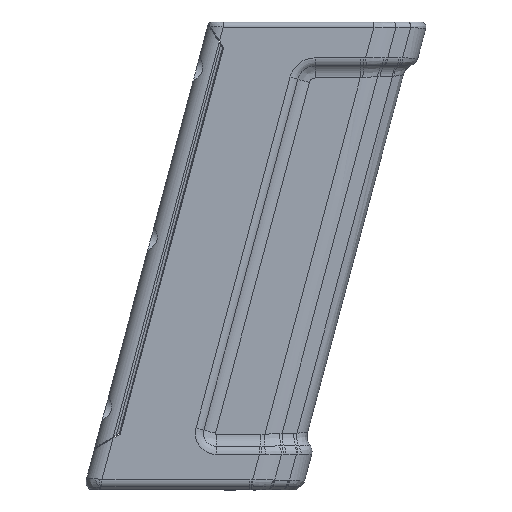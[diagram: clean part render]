
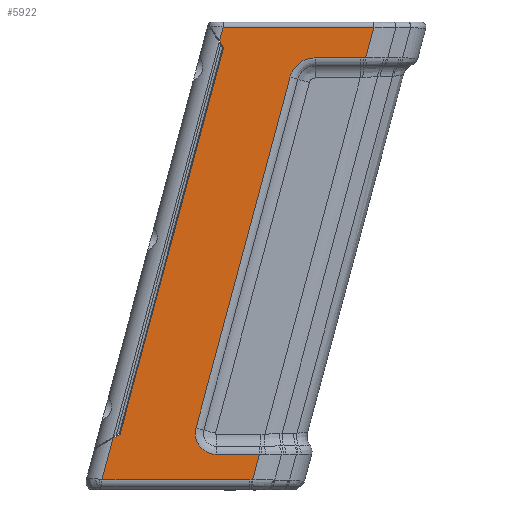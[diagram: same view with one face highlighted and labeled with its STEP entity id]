
A CAD part, left-side view. The second image highlights one B-rep face of the part: STEP entity #5922.
In plain terms, the highlighted planar face has unit normal (-1, 0, 0).
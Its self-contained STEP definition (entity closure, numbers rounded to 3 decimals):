
#297=PLANE('',#6416);
#440=FACE_OUTER_BOUND('',#836,.T.);
#836=EDGE_LOOP('',(#4337,#4338,#4339,#4340,#4341,#4342,#4343,#4344,#4345,
#4346,#4347,#4348,#4349,#4350,#4351,#4352,#4353,#4354));
#1217=LINE('',#9080,#1559);
#1229=LINE('',#9156,#1571);
#1238=LINE('',#9196,#1580);
#1246=LINE('',#9251,#1588);
#1247=LINE('',#9253,#1589);
#1248=LINE('',#9265,#1590);
#1249=LINE('',#9267,#1591);
#1250=LINE('',#9271,#1592);
#1251=LINE('',#9275,#1593);
#1252=LINE('',#9287,#1594);
#1253=LINE('',#9288,#1595);
#1254=LINE('',#9289,#1596);
#1559=VECTOR('',#7221,10.);
#1571=VECTOR('',#7247,10.);
#1580=VECTOR('',#7264,10.);
#1588=VECTOR('',#7294,10.);
#1589=VECTOR('',#7295,10.);
#1590=VECTOR('',#7296,10.);
#1591=VECTOR('',#7297,10.);
#1592=VECTOR('',#7300,10.);
#1593=VECTOR('',#7303,10.);
#1594=VECTOR('',#7304,10.);
#1595=VECTOR('',#7305,10.);
#1596=VECTOR('',#7306,10.);
#1888=CIRCLE('',#6417,4.172);
#1889=CIRCLE('',#6418,5.172);
#2124=B_SPLINE_CURVE_WITH_KNOTS('',3,(#9255,#9256,#9257,#9258),
 .UNSPECIFIED.,.F.,.F.,(4,4),(0.,0.029),.UNSPECIFIED.);
#2125=B_SPLINE_CURVE_WITH_KNOTS('',3,(#9260,#9261,#9262,#9263),
 .UNSPECIFIED.,.F.,.F.,(4,4),(0.,0.027),.UNSPECIFIED.);
#2126=B_SPLINE_CURVE_WITH_KNOTS('',3,(#9277,#9278,#9279,#9280),
 .UNSPECIFIED.,.F.,.F.,(4,4),(-0.063,0.),.UNSPECIFIED.);
#2127=B_SPLINE_CURVE_WITH_KNOTS('',3,(#9282,#9283,#9284,#9285),
 .UNSPECIFIED.,.F.,.F.,(4,4),(-0.045,0.),
 .UNSPECIFIED.);
#2499=VERTEX_POINT('',#9077);
#2500=VERTEX_POINT('',#9079);
#2518=VERTEX_POINT('',#9155);
#2529=VERTEX_POINT('',#9195);
#2538=VERTEX_POINT('',#9244);
#2540=VERTEX_POINT('',#9250);
#2541=VERTEX_POINT('',#9252);
#2542=VERTEX_POINT('',#9254);
#2543=VERTEX_POINT('',#9259);
#2544=VERTEX_POINT('',#9264);
#2545=VERTEX_POINT('',#9266);
#2546=VERTEX_POINT('',#9268);
#2547=VERTEX_POINT('',#9270);
#2548=VERTEX_POINT('',#9272);
#2549=VERTEX_POINT('',#9274);
#2550=VERTEX_POINT('',#9276);
#2551=VERTEX_POINT('',#9281);
#2552=VERTEX_POINT('',#9286);
#3144=EDGE_CURVE('',#2500,#2499,#1217,.T.);
#3165=EDGE_CURVE('',#2518,#2500,#1229,.T.);
#3178=EDGE_CURVE('',#2499,#2529,#1238,.F.);
#3194=EDGE_CURVE('',#2540,#2529,#1246,.T.);
#3195=EDGE_CURVE('',#2541,#2540,#1247,.T.);
#3196=EDGE_CURVE('',#2542,#2541,#2124,.T.);
#3197=EDGE_CURVE('',#2543,#2542,#2125,.T.);
#3198=EDGE_CURVE('',#2544,#2543,#1248,.T.);
#3199=EDGE_CURVE('',#2545,#2544,#1249,.T.);
#3200=EDGE_CURVE('',#2546,#2545,#1888,.T.);
#3201=EDGE_CURVE('',#2547,#2546,#1250,.T.);
#3202=EDGE_CURVE('',#2548,#2547,#1889,.T.);
#3203=EDGE_CURVE('',#2549,#2548,#1251,.T.);
#3204=EDGE_CURVE('',#2550,#2549,#2126,.T.);
#3205=EDGE_CURVE('',#2551,#2550,#2127,.T.);
#3206=EDGE_CURVE('',#2552,#2551,#1252,.T.);
#3207=EDGE_CURVE('',#2538,#2552,#1253,.T.);
#3208=EDGE_CURVE('',#2518,#2538,#1254,.T.);
#4337=ORIENTED_EDGE('',*,*,#3165,.T.);
#4338=ORIENTED_EDGE('',*,*,#3144,.T.);
#4339=ORIENTED_EDGE('',*,*,#3178,.T.);
#4340=ORIENTED_EDGE('',*,*,#3194,.F.);
#4341=ORIENTED_EDGE('',*,*,#3195,.F.);
#4342=ORIENTED_EDGE('',*,*,#3196,.F.);
#4343=ORIENTED_EDGE('',*,*,#3197,.F.);
#4344=ORIENTED_EDGE('',*,*,#3198,.F.);
#4345=ORIENTED_EDGE('',*,*,#3199,.F.);
#4346=ORIENTED_EDGE('',*,*,#3200,.F.);
#4347=ORIENTED_EDGE('',*,*,#3201,.F.);
#4348=ORIENTED_EDGE('',*,*,#3202,.F.);
#4349=ORIENTED_EDGE('',*,*,#3203,.F.);
#4350=ORIENTED_EDGE('',*,*,#3204,.F.);
#4351=ORIENTED_EDGE('',*,*,#3205,.F.);
#4352=ORIENTED_EDGE('',*,*,#3206,.F.);
#4353=ORIENTED_EDGE('',*,*,#3207,.F.);
#4354=ORIENTED_EDGE('',*,*,#3208,.F.);
#5922=ADVANCED_FACE('',(#440),#297,.F.);
#6416=AXIS2_PLACEMENT_3D('',#9249,#7292,#7293);
#6417=AXIS2_PLACEMENT_3D('',#9269,#7298,#7299);
#6418=AXIS2_PLACEMENT_3D('',#9273,#7301,#7302);
#7221=DIRECTION('',(0.,0.259,-0.966));
#7247=DIRECTION('',(0.,-0.537,-0.844));
#7264=DIRECTION('',(0.,-0.86,0.51));
#7292=DIRECTION('center_axis',(1.,0.,0.));
#7293=DIRECTION('ref_axis',(0.,1.,0.));
#7294=DIRECTION('',(0.,-0.259,0.966));
#7295=DIRECTION('',(0.,1.,0.));
#7296=DIRECTION('',(0.,0.259,-0.966));
#7297=DIRECTION('',(0.,-1.,0.));
#7298=DIRECTION('center_axis',(-1.,0.,0.));
#7299=DIRECTION('ref_axis',(0.,0.793,-0.609));
#7300=DIRECTION('',(0.,0.259,-0.966));
#7301=DIRECTION('center_axis',(-1.,0.,0.));
#7302=DIRECTION('ref_axis',(0.,0.609,0.793));
#7303=DIRECTION('',(0.,1.,0.));
#7304=DIRECTION('',(0.,0.259,-0.966));
#7305=DIRECTION('',(0.,-1.,0.));
#7306=DIRECTION('',(0.,-0.259,0.966));
#9077=CARTESIAN_POINT('',(8.281,19.826,-74.034));
#9079=CARTESIAN_POINT('',(8.281,-0.788,2.901));
#9080=CARTESIAN_POINT('',(8.281,11.023,-41.18));
#9155=CARTESIAN_POINT('',(8.281,0.048,4.215));
#9156=CARTESIAN_POINT('',(8.281,-2.855,-0.348));
#9195=CARTESIAN_POINT('',(8.281,21.239,-74.872));
#9196=CARTESIAN_POINT('',(8.281,1.91,-63.414));
#9244=CARTESIAN_POINT('',(8.281,-0.689,6.965));
#9249=CARTESIAN_POINT('Origin',(8.281,2.424,-8.271));
#9250=CARTESIAN_POINT('',(8.281,23.442,-83.093));
#9251=CARTESIAN_POINT('',(8.281,3.465,-8.538));
#9252=CARTESIAN_POINT('',(8.281,-6.,-83.093));
#9253=CARTESIAN_POINT('',(8.281,-2.868,-83.093));
#9254=CARTESIAN_POINT('',(8.281,-6.289,-83.09));
#9255=CARTESIAN_POINT('Ctrl Pts',(8.281,-6.289,-83.09));
#9256=CARTESIAN_POINT('Ctrl Pts',(8.281,-6.192,-83.092));
#9257=CARTESIAN_POINT('Ctrl Pts',(8.281,-6.096,-83.093));
#9258=CARTESIAN_POINT('Ctrl Pts',(8.281,-6.,-83.093));
#9259=CARTESIAN_POINT('',(8.281,-6.56,-83.08));
#9260=CARTESIAN_POINT('Ctrl Pts',(8.281,-6.56,-83.08));
#9261=CARTESIAN_POINT('Ctrl Pts',(8.281,-6.47,-83.085));
#9262=CARTESIAN_POINT('Ctrl Pts',(8.281,-6.379,-83.089));
#9263=CARTESIAN_POINT('Ctrl Pts',(8.281,-6.289,-83.09));
#9264=CARTESIAN_POINT('',(8.281,-7.897,-78.093));
#9265=CARTESIAN_POINT('',(8.281,-28.055,-2.863));
#9266=CARTESIAN_POINT('',(8.281,0.694,-78.093));
#9267=CARTESIAN_POINT('',(8.281,-2.358,-78.093));
#9268=CARTESIAN_POINT('',(8.281,4.723,-72.841));
#9269=CARTESIAN_POINT('Origin',(8.281,0.694,-73.921));
#9270=CARTESIAN_POINT('',(8.281,-13.988,-3.011));
#9271=CARTESIAN_POINT('',(8.281,-13.251,-5.762));
#9272=CARTESIAN_POINT('',(8.281,-18.983,0.822));
#9273=CARTESIAN_POINT('Origin',(8.281,-18.983,-4.349));
#9274=CARTESIAN_POINT('',(8.281,-27.97,0.822));
#9275=CARTESIAN_POINT('',(8.281,-2.358,0.822));
#9276=CARTESIAN_POINT('',(8.281,-28.602,0.832));
#9277=CARTESIAN_POINT('Ctrl Pts',(8.281,-28.602,0.832));
#9278=CARTESIAN_POINT('Ctrl Pts',(8.281,-28.391,0.826));
#9279=CARTESIAN_POINT('Ctrl Pts',(8.281,-28.181,0.822));
#9280=CARTESIAN_POINT('Ctrl Pts',(8.281,-27.97,0.822));
#9281=CARTESIAN_POINT('',(8.281,-29.051,0.858));
#9282=CARTESIAN_POINT('Ctrl Pts',(8.281,-29.051,0.858));
#9283=CARTESIAN_POINT('Ctrl Pts',(8.281,-28.902,0.846));
#9284=CARTESIAN_POINT('Ctrl Pts',(8.281,-28.752,0.837));
#9285=CARTESIAN_POINT('Ctrl Pts',(8.281,-28.602,0.832));
#9286=CARTESIAN_POINT('',(8.281,-30.688,6.965));
#9287=CARTESIAN_POINT('',(8.281,-28.055,-2.863));
#9288=CARTESIAN_POINT('',(8.281,-8.445,6.965));
#9289=CARTESIAN_POINT('',(8.281,3.465,-8.538));
